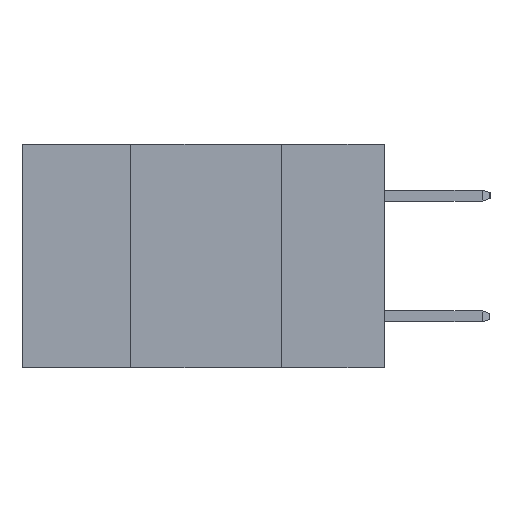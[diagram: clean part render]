
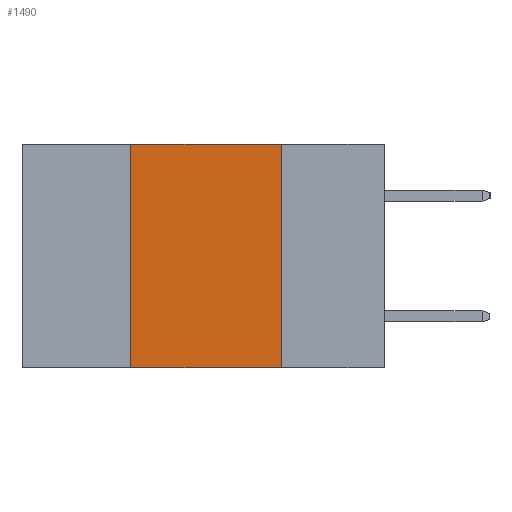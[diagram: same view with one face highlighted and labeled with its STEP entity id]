
A CAD part, left-side view. The second image highlights one B-rep face of the part: STEP entity #1490.
In plain terms, the highlighted planar face has unit normal (-1, 0, 0).
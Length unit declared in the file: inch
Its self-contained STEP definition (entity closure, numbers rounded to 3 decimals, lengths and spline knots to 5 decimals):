
#379 = DIRECTION ( 'NONE',  ( 0., -1., 0. ) ) ;
#436 = CARTESIAN_POINT ( 'NONE',  ( 0., 0.6, 0. ) ) ;
#1119 = CARTESIAN_POINT ( 'NONE',  ( 0., 0.6, 0. ) ) ;
#1172 = PLANE ( 'NONE',  #3271 ) ;
#1225 = DIRECTION ( 'NONE',  ( 0., 0., -1. ) ) ;
#1274 = VECTOR ( 'NONE', #3551, 39.37008 ) ;
#1292 = DIRECTION ( 'NONE',  ( 1., 0., 0. ) ) ;
#1490 = ADVANCED_FACE ( 'NONE', ( #9373 ), #1172, .F. ) ;
#2724 = EDGE_CURVE ( 'NONE', #9366, #13452, #4176, .T. ) ;
#3153 = EDGE_CURVE ( 'NONE', #4759, #13452, #13426, .T. ) ;
#3271 = AXIS2_PLACEMENT_3D ( 'NONE', #1119, #1292, #1225 ) ;
#3551 = DIRECTION ( 'NONE',  ( 0., -1., 0. ) ) ;
#4176 = LINE ( 'NONE', #5109, #1274 ) ;
#4266 = ORIENTED_EDGE ( 'NONE', *, *, #3153, .F. ) ;
#4295 = DIRECTION ( 'NONE',  ( 0., 0., 1. ) ) ;
#4735 = ORIENTED_EDGE ( 'NONE', *, *, #6352, .F. ) ;
#4759 = VERTEX_POINT ( 'NONE', #13029 ) ;
#5109 = CARTESIAN_POINT ( 'NONE',  ( 0., 0.6, -0.37 ) ) ;
#5519 = EDGE_LOOP ( 'NONE', ( #4266, #8205, #4735, #7772 ) ) ;
#5926 = CARTESIAN_POINT ( 'NONE',  ( 0., 0.17, -0.37 ) ) ;
#6188 = LINE ( 'NONE', #9033, #8769 ) ;
#6352 = EDGE_CURVE ( 'NONE', #9366, #14011, #6188, .T. ) ;
#7113 = CARTESIAN_POINT ( 'NONE',  ( 0., 0.17, 0. ) ) ;
#7318 = DIRECTION ( 'NONE',  ( 0., 0., -1. ) ) ;
#7767 = VECTOR ( 'NONE', #7318, 39.37008 ) ;
#7772 = ORIENTED_EDGE ( 'NONE', *, *, #2724, .T. ) ;
#8205 = ORIENTED_EDGE ( 'NONE', *, *, #10891, .F. ) ;
#8769 = VECTOR ( 'NONE', #4295, 39.37008 ) ;
#9033 = CARTESIAN_POINT ( 'NONE',  ( 0., 0.42, 0. ) ) ;
#9366 = VERTEX_POINT ( 'NONE', #11598 ) ;
#9373 = FACE_OUTER_BOUND ( 'NONE', #5519, .T. ) ;
#10209 = CARTESIAN_POINT ( 'NONE',  ( 0., 0.42, 0. ) ) ;
#10891 = EDGE_CURVE ( 'NONE', #14011, #4759, #13904, .T. ) ;
#11212 = VECTOR ( 'NONE', #379, 39.37008 ) ;
#11598 = CARTESIAN_POINT ( 'NONE',  ( 0., 0.42, -0.37 ) ) ;
#13029 = CARTESIAN_POINT ( 'NONE',  ( 0., 0.17, 0. ) ) ;
#13426 = LINE ( 'NONE', #7113, #7767 ) ;
#13452 = VERTEX_POINT ( 'NONE', #5926 ) ;
#13904 = LINE ( 'NONE', #436, #11212 ) ;
#14011 = VERTEX_POINT ( 'NONE', #10209 ) ;
